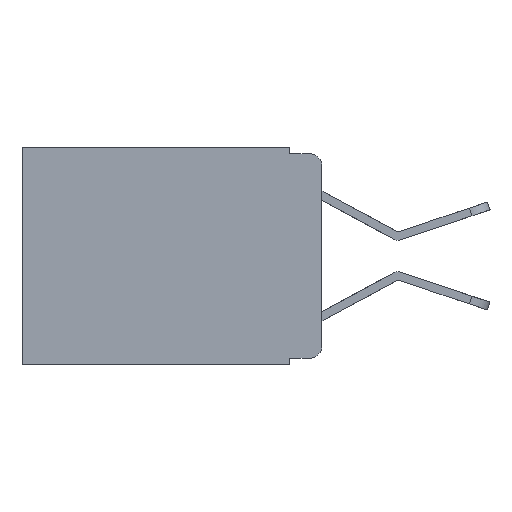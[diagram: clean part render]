
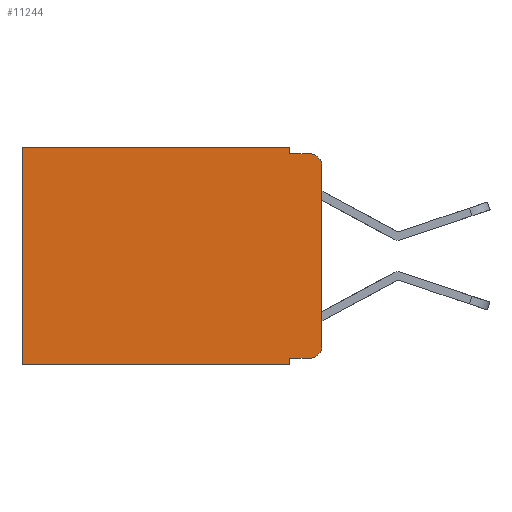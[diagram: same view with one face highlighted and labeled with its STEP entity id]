
A CAD part, left-side view. The second image highlights one B-rep face of the part: STEP entity #11244.
In plain terms, the highlighted planar face has unit normal (-1, 0, 0).
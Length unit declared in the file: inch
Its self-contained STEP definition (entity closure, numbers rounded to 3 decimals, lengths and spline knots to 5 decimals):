
#317 = CARTESIAN_POINT ( 'NONE',  ( 0.298, 0.051, 0. ) ) ;
#485 = ORIENTED_EDGE ( 'NONE', *, *, #14959, .T. ) ;
#570 = VERTEX_POINT ( 'NONE', #13887 ) ;
#678 = CIRCLE ( 'NONE', #8771, 0.02 ) ;
#879 = EDGE_CURVE ( 'NONE', #6978, #16830, #7446, .T. ) ;
#911 = ORIENTED_EDGE ( 'NONE', *, *, #13497, .F. ) ;
#1099 = LINE ( 'NONE', #14733, #4898 ) ;
#1339 = CARTESIAN_POINT ( 'NONE',  ( 0.298, 0.051, -0.343 ) ) ;
#1388 = VERTEX_POINT ( 'NONE', #5936 ) ;
#2111 = EDGE_CURVE ( 'NONE', #13687, #5412, #17258, .T. ) ;
#2435 = ORIENTED_EDGE ( 'NONE', *, *, #2111, .T. ) ;
#2460 = VERTEX_POINT ( 'NONE', #3904 ) ;
#2552 = DIRECTION ( 'NONE',  ( 0., 0., -1. ) ) ;
#2589 = VECTOR ( 'NONE', #9942, 39.37008 ) ;
#2673 = CARTESIAN_POINT ( 'NONE',  ( 0.298, 0.051, 0. ) ) ;
#2681 = ORIENTED_EDGE ( 'NONE', *, *, #4748, .F. ) ;
#2964 = DIRECTION ( 'NONE',  ( 0., 0., -1. ) ) ;
#3393 = CARTESIAN_POINT ( 'NONE',  ( 0.298, 0.051, 0. ) ) ;
#3773 = VECTOR ( 'NONE', #16010, 39.37008 ) ;
#3904 = CARTESIAN_POINT ( 'NONE',  ( 0.298, 0.051, -0.01 ) ) ;
#3932 = CARTESIAN_POINT ( 'NONE',  ( 0.298, 0., 0. ) ) ;
#4748 = EDGE_CURVE ( 'NONE', #16830, #13237, #6908, .T. ) ;
#4898 = VECTOR ( 'NONE', #2964, 39.37008 ) ;
#5163 = CARTESIAN_POINT ( 'NONE',  ( 0.298, 0.051, -0.333 ) ) ;
#5283 = PLANE ( 'NONE',  #9677 ) ;
#5412 = VERTEX_POINT ( 'NONE', #12357 ) ;
#5464 = CARTESIAN_POINT ( 'NONE',  ( 0.298, 0.473, -0.343 ) ) ;
#5936 = CARTESIAN_POINT ( 'NONE',  ( 0.298, 0., -0.03 ) ) ;
#6306 = EDGE_CURVE ( 'NONE', #6978, #13687, #13386, .T. ) ;
#6374 = AXIS2_PLACEMENT_3D ( 'NONE', #16974, #16943, #10770 ) ;
#6608 = DIRECTION ( 'NONE',  ( 1., 0., 0. ) ) ;
#6624 = VECTOR ( 'NONE', #8103, 39.37008 ) ;
#6643 = CARTESIAN_POINT ( 'NONE',  ( 0.298, 0.02, -0.03 ) ) ;
#6908 = LINE ( 'NONE', #12212, #3773 ) ;
#6978 = VERTEX_POINT ( 'NONE', #5163 ) ;
#7446 = LINE ( 'NONE', #2673, #6624 ) ;
#7580 = ORIENTED_EDGE ( 'NONE', *, *, #9298, .T. ) ;
#7650 = EDGE_LOOP ( 'NONE', ( #10792, #10333, #10182, #911, #7580, #485, #2681, #11193, #14991, #2435 ) ) ;
#7968 = DIRECTION ( 'NONE',  ( 0., 0., -1. ) ) ;
#8042 = LINE ( 'NONE', #3932, #10735 ) ;
#8103 = DIRECTION ( 'NONE',  ( 0., 0., -1. ) ) ;
#8444 = DIRECTION ( 'NONE',  ( 0., 1., 0. ) ) ;
#8682 = VECTOR ( 'NONE', #8444, 39.37008 ) ;
#8771 = AXIS2_PLACEMENT_3D ( 'NONE', #6643, #15654, #7968 ) ;
#9191 = CARTESIAN_POINT ( 'NONE',  ( 0.298, 0., 0. ) ) ;
#9197 = EDGE_CURVE ( 'NONE', #2460, #12241, #13298, .T. ) ;
#9258 = LINE ( 'NONE', #317, #2589 ) ;
#9298 = EDGE_CURVE ( 'NONE', #10978, #570, #15082, .T. ) ;
#9526 = CARTESIAN_POINT ( 'NONE',  ( 0.298, 0.051, -0.01 ) ) ;
#9626 = EDGE_CURVE ( 'NONE', #1388, #12241, #678, .T. ) ;
#9677 = AXIS2_PLACEMENT_3D ( 'NONE', #9191, #6608, #15620 ) ;
#9942 = DIRECTION ( 'NONE',  ( 0., 0., -1. ) ) ;
#10182 = ORIENTED_EDGE ( 'NONE', *, *, #9197, .F. ) ;
#10191 = DIRECTION ( 'NONE',  ( 0., -1., 0. ) ) ;
#10333 = ORIENTED_EDGE ( 'NONE', *, *, #9626, .T. ) ;
#10735 = VECTOR ( 'NONE', #2552, 39.37008 ) ;
#10770 = DIRECTION ( 'NONE',  ( 0., 0., -1. ) ) ;
#10792 = ORIENTED_EDGE ( 'NONE', *, *, #13140, .F. ) ;
#10978 = VERTEX_POINT ( 'NONE', #3393 ) ;
#11193 = ORIENTED_EDGE ( 'NONE', *, *, #879, .F. ) ;
#11244 = ADVANCED_FACE ( 'NONE', ( #16209 ), #5283, .F. ) ;
#12212 = CARTESIAN_POINT ( 'NONE',  ( 0.298, 0., -0.343 ) ) ;
#12241 = VERTEX_POINT ( 'NONE', #16201 ) ;
#12357 = CARTESIAN_POINT ( 'NONE',  ( 0.298, 0., -0.313 ) ) ;
#13004 = VECTOR ( 'NONE', #10191, 39.37008 ) ;
#13140 = EDGE_CURVE ( 'NONE', #1388, #5412, #8042, .T. ) ;
#13214 = CARTESIAN_POINT ( 'NONE',  ( 0.298, 0.02, -0.333 ) ) ;
#13237 = VERTEX_POINT ( 'NONE', #5464 ) ;
#13298 = LINE ( 'NONE', #9526, #16281 ) ;
#13386 = LINE ( 'NONE', #16541, #13004 ) ;
#13497 = EDGE_CURVE ( 'NONE', #10978, #2460, #9258, .T. ) ;
#13687 = VERTEX_POINT ( 'NONE', #13214 ) ;
#13887 = CARTESIAN_POINT ( 'NONE',  ( 0.298, 0.473, 0. ) ) ;
#14733 = CARTESIAN_POINT ( 'NONE',  ( 0.298, 0.473, 0. ) ) ;
#14959 = EDGE_CURVE ( 'NONE', #570, #13237, #1099, .T. ) ;
#14991 = ORIENTED_EDGE ( 'NONE', *, *, #6306, .T. ) ;
#15082 = LINE ( 'NONE', #16099, #8682 ) ;
#15620 = DIRECTION ( 'NONE',  ( 0., 0., -1. ) ) ;
#15654 = DIRECTION ( 'NONE',  ( -1., 0., 0. ) ) ;
#16010 = DIRECTION ( 'NONE',  ( 0., 1., 0. ) ) ;
#16099 = CARTESIAN_POINT ( 'NONE',  ( 0.298, 0., 0. ) ) ;
#16201 = CARTESIAN_POINT ( 'NONE',  ( 0.298, 0.02, -0.01 ) ) ;
#16209 = FACE_OUTER_BOUND ( 'NONE', #7650, .T. ) ;
#16281 = VECTOR ( 'NONE', #17181, 39.37008 ) ;
#16541 = CARTESIAN_POINT ( 'NONE',  ( 0.298, 0.051, -0.333 ) ) ;
#16830 = VERTEX_POINT ( 'NONE', #1339 ) ;
#16943 = DIRECTION ( 'NONE',  ( -1., 0., 0. ) ) ;
#16974 = CARTESIAN_POINT ( 'NONE',  ( 0.298, 0.02, -0.313 ) ) ;
#17181 = DIRECTION ( 'NONE',  ( 0., -1., 0. ) ) ;
#17258 = CIRCLE ( 'NONE', #6374, 0.02 ) ;
